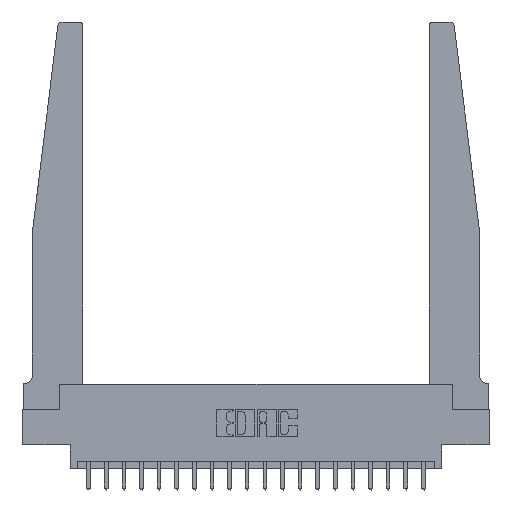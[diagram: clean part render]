
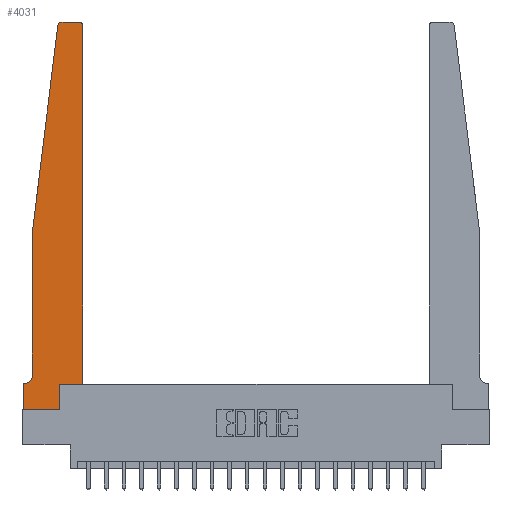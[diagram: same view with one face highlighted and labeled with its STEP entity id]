
A CAD part, top view. The second image highlights one B-rep face of the part: STEP entity #4031.
In plain terms, the highlighted planar face has unit normal (0, 0, 1).
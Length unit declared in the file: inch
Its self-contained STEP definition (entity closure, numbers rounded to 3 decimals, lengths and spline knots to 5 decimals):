
#222 = CARTESIAN_POINT ( 'NONE',  ( 0., 0., 0.37 ) ) ;
#506 = ORIENTED_EDGE ( 'NONE', *, *, #15833, .T. ) ;
#629 = AXIS2_PLACEMENT_3D ( 'NONE', #17220, #12062, #3936 ) ;
#813 = LINE ( 'NONE', #15930, #9282 ) ;
#874 = CARTESIAN_POINT ( 'NONE',  ( 0.425, 0.18, 0.37 ) ) ;
#1160 = CARTESIAN_POINT ( 'NONE',  ( 0.2605, 0.18, 0.37 ) ) ;
#1329 = DIRECTION ( 'NONE',  ( 1., 0., 0. ) ) ;
#1665 = CARTESIAN_POINT ( 'NONE',  ( 0., 0., 0.37 ) ) ;
#1907 = CARTESIAN_POINT ( 'NONE',  ( 0.27653, 2.72, 0.37 ) ) ;
#1915 = CARTESIAN_POINT ( 'NONE',  ( 0.24675, 2.72367, 0.37 ) ) ;
#1952 = EDGE_CURVE ( 'NONE', #18434, #17710, #4030, .T. ) ;
#1961 = DIRECTION ( 'NONE',  ( 1., 0., 0. ) ) ;
#2020 = ORIENTED_EDGE ( 'NONE', *, *, #5845, .T. ) ;
#2211 = CARTESIAN_POINT ( 'NONE',  ( 0.2605, 0.18, 0.37 ) ) ;
#2319 = VECTOR ( 'NONE', #9504, 39.37008 ) ;
#2386 = VERTEX_POINT ( 'NONE', #1915 ) ;
#2575 = CARTESIAN_POINT ( 'NONE',  ( 0.065, 0.2375, 0.37 ) ) ;
#3338 = CARTESIAN_POINT ( 'NONE',  ( 0., 0., 0.37 ) ) ;
#3502 = PLANE ( 'NONE',  #20154 ) ;
#3729 = DIRECTION ( 'NONE',  ( 0., 1., 0. ) ) ;
#3921 = DIRECTION ( 'NONE',  ( 1., 0., 0. ) ) ;
#3936 = DIRECTION ( 'NONE',  ( -1., 0., 0. ) ) ;
#3939 = CARTESIAN_POINT ( 'NONE',  ( 0.425, 0.18, 0.37 ) ) ;
#4019 = CARTESIAN_POINT ( 'NONE',  ( 0.065, 1.25, 0.37 ) ) ;
#4030 = LINE ( 'NONE', #2211, #17719 ) ;
#4031 = ADVANCED_FACE ( 'NONE', ( #5221 ), #3502, .T. ) ;
#4805 = EDGE_CURVE ( 'NONE', #6368, #14515, #18740, .T. ) ;
#5134 = AXIS2_PLACEMENT_3D ( 'NONE', #1907, #13654, #3921 ) ;
#5221 = FACE_OUTER_BOUND ( 'NONE', #12617, .T. ) ;
#5352 = VERTEX_POINT ( 'NONE', #4019 ) ;
#5845 = EDGE_CURVE ( 'NONE', #17710, #6368, #12324, .T. ) ;
#5984 = CIRCLE ( 'NONE', #8082, 0.03 ) ;
#6368 = VERTEX_POINT ( 'NONE', #8773 ) ;
#7217 = EDGE_CURVE ( 'NONE', #5352, #15963, #8174, .T. ) ;
#7272 = ORIENTED_EDGE ( 'NONE', *, *, #12096, .T. ) ;
#7320 = EDGE_CURVE ( 'NONE', #15963, #10268, #13734, .T. ) ;
#7410 = DIRECTION ( 'NONE',  ( -0.122, -0.992, 0. ) ) ;
#7539 = CARTESIAN_POINT ( 'NONE',  ( 0.015, 0.1875, 0.37 ) ) ;
#8021 = CARTESIAN_POINT ( 'NONE',  ( 0.395, 2.72, 0.37 ) ) ;
#8082 = AXIS2_PLACEMENT_3D ( 'NONE', #8021, #9543, #1329 ) ;
#8174 = LINE ( 'NONE', #15071, #14741 ) ;
#8773 = CARTESIAN_POINT ( 'NONE',  ( 0.425, 0.18, 0.37 ) ) ;
#8893 = DIRECTION ( 'NONE',  ( 0., 1., 0. ) ) ;
#9173 = EDGE_CURVE ( 'NONE', #14515, #18760, #5984, .T. ) ;
#9282 = VECTOR ( 'NONE', #7410, 39.37008 ) ;
#9504 = DIRECTION ( 'NONE',  ( -1., 0., 0. ) ) ;
#9543 = DIRECTION ( 'NONE',  ( 0., 0., 1. ) ) ;
#10146 = CARTESIAN_POINT ( 'NONE',  ( 0.425, 2.72, 0.37 ) ) ;
#10205 = VECTOR ( 'NONE', #1961, 39.37008 ) ;
#10268 = VERTEX_POINT ( 'NONE', #7539 ) ;
#10310 = CARTESIAN_POINT ( 'NONE',  ( 0., 0.1875, 0.37 ) ) ;
#11381 = ORIENTED_EDGE ( 'NONE', *, *, #16514, .T. ) ;
#11686 = DIRECTION ( 'NONE',  ( -1., 0., 0. ) ) ;
#11798 = CARTESIAN_POINT ( 'NONE',  ( 0.25, 2.75, 0.37 ) ) ;
#11832 = DIRECTION ( 'NONE',  ( 0., 0., 1. ) ) ;
#11952 = CARTESIAN_POINT ( 'NONE',  ( 0.395, 2.75, 0.37 ) ) ;
#12062 = DIRECTION ( 'NONE',  ( 0., 0., -1. ) ) ;
#12096 = EDGE_CURVE ( 'NONE', #14893, #2386, #12365, .T. ) ;
#12141 = DIRECTION ( 'NONE',  ( 1., 0., 0. ) ) ;
#12216 = DIRECTION ( 'NONE',  ( 1., 0., 0. ) ) ;
#12324 = LINE ( 'NONE', #874, #19286 ) ;
#12365 = CIRCLE ( 'NONE', #5134, 0.03 ) ;
#12617 = EDGE_LOOP ( 'NONE', ( #17496, #7272, #19444, #20332, #17253, #18745, #11381, #506, #15900, #2020, #16533, #21165 ) ) ;
#13005 = DIRECTION ( 'NONE',  ( 0., -1., 0. ) ) ;
#13654 = DIRECTION ( 'NONE',  ( 0., 0., 1. ) ) ;
#13734 = CIRCLE ( 'NONE', #629, 0.05 ) ;
#13927 = VERTEX_POINT ( 'NONE', #3338 ) ;
#14127 = CARTESIAN_POINT ( 'NONE',  ( 0., 0.1875, 0.37 ) ) ;
#14236 = LINE ( 'NONE', #20861, #2319 ) ;
#14492 = DIRECTION ( 'NONE',  ( 0., -1., 0. ) ) ;
#14515 = VERTEX_POINT ( 'NONE', #10146 ) ;
#14741 = VECTOR ( 'NONE', #14492, 39.37008 ) ;
#14893 = VERTEX_POINT ( 'NONE', #17004 ) ;
#15011 = LINE ( 'NONE', #11798, #19848 ) ;
#15071 = CARTESIAN_POINT ( 'NONE',  ( 0.065, 1.25, 0.37 ) ) ;
#15370 = VECTOR ( 'NONE', #13005, 39.37008 ) ;
#15803 = EDGE_CURVE ( 'NONE', #18760, #14893, #15011, .T. ) ;
#15833 = EDGE_CURVE ( 'NONE', #13927, #18434, #16755, .T. ) ;
#15900 = ORIENTED_EDGE ( 'NONE', *, *, #1952, .T. ) ;
#15930 = CARTESIAN_POINT ( 'NONE',  ( 0.065, 1.25, 0.37 ) ) ;
#15963 = VERTEX_POINT ( 'NONE', #2575 ) ;
#16514 = EDGE_CURVE ( 'NONE', #17176, #13927, #19266, .T. ) ;
#16533 = ORIENTED_EDGE ( 'NONE', *, *, #4805, .T. ) ;
#16755 = LINE ( 'NONE', #222, #10205 ) ;
#17004 = CARTESIAN_POINT ( 'NONE',  ( 0.27653, 2.75, 0.37 ) ) ;
#17176 = VERTEX_POINT ( 'NONE', #14127 ) ;
#17220 = CARTESIAN_POINT ( 'NONE',  ( 0.015, 0.2375, 0.37 ) ) ;
#17253 = ORIENTED_EDGE ( 'NONE', *, *, #7320, .T. ) ;
#17496 = ORIENTED_EDGE ( 'NONE', *, *, #15803, .T. ) ;
#17710 = VERTEX_POINT ( 'NONE', #1160 ) ;
#17719 = VECTOR ( 'NONE', #8893, 39.37008 ) ;
#17775 = VECTOR ( 'NONE', #3729, 39.37008 ) ;
#18023 = EDGE_CURVE ( 'NONE', #10268, #17176, #14236, .T. ) ;
#18434 = VERTEX_POINT ( 'NONE', #18864 ) ;
#18740 = LINE ( 'NONE', #3939, #17775 ) ;
#18745 = ORIENTED_EDGE ( 'NONE', *, *, #18023, .T. ) ;
#18760 = VERTEX_POINT ( 'NONE', #11952 ) ;
#18864 = CARTESIAN_POINT ( 'NONE',  ( 0.2605, 0., 0.37 ) ) ;
#19266 = LINE ( 'NONE', #1665, #15370 ) ;
#19286 = VECTOR ( 'NONE', #12216, 39.37008 ) ;
#19444 = ORIENTED_EDGE ( 'NONE', *, *, #20102, .T. ) ;
#19848 = VECTOR ( 'NONE', #11686, 39.37008 ) ;
#20102 = EDGE_CURVE ( 'NONE', #2386, #5352, #813, .T. ) ;
#20154 = AXIS2_PLACEMENT_3D ( 'NONE', #10310, #11832, #12141 ) ;
#20332 = ORIENTED_EDGE ( 'NONE', *, *, #7217, .T. ) ;
#20861 = CARTESIAN_POINT ( 'NONE',  ( 0.065, 0.1875, 0.37 ) ) ;
#21165 = ORIENTED_EDGE ( 'NONE', *, *, #9173, .T. ) ;
